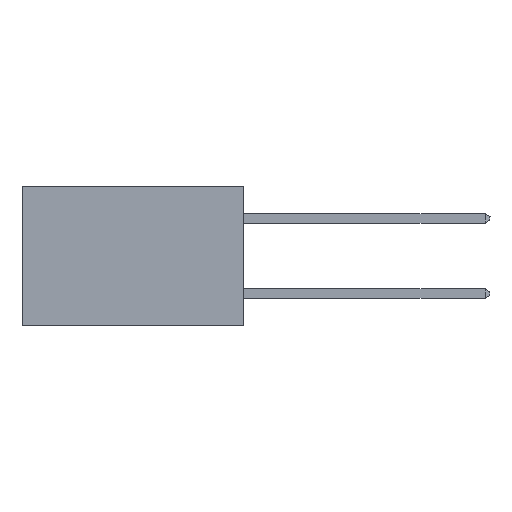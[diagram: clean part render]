
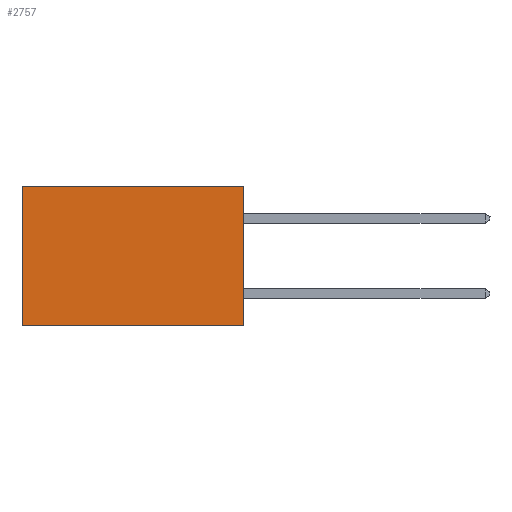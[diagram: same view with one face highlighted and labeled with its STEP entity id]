
A CAD part, left-side view. The second image highlights one B-rep face of the part: STEP entity #2757.
In plain terms, the highlighted planar face has unit normal (-1, 0, 0).
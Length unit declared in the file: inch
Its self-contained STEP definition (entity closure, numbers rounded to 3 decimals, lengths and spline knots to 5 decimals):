
#101 = EDGE_CURVE ( 'NONE', #1082, #926, #6169, .T. ) ;
#853 = LINE ( 'NONE', #5399, #7291 ) ;
#926 = VERTEX_POINT ( 'NONE', #7003 ) ;
#1082 = VERTEX_POINT ( 'NONE', #3588 ) ;
#1115 = AXIS2_PLACEMENT_3D ( 'NONE', #5558, #6310, #5442 ) ;
#1515 = DIRECTION ( 'NONE',  ( 0., 0., -1. ) ) ;
#1756 = EDGE_CURVE ( 'NONE', #5937, #1082, #5213, .T. ) ;
#1921 = EDGE_CURVE ( 'NONE', #5937, #4105, #853, .T. ) ;
#2757 = ADVANCED_FACE ( 'NONE', ( #6491 ), #5560, .F. ) ;
#2960 = VECTOR ( 'NONE', #7861, 39.37008 ) ;
#3369 = CARTESIAN_POINT ( 'NONE',  ( 0.277, 0., -0.37 ) ) ;
#3583 = VECTOR ( 'NONE', #5382, 39.37008 ) ;
#3588 = CARTESIAN_POINT ( 'NONE',  ( 0.277, 0., -0.37 ) ) ;
#3612 = ORIENTED_EDGE ( 'NONE', *, *, #7612, .T. ) ;
#3624 = ORIENTED_EDGE ( 'NONE', *, *, #1756, .F. ) ;
#3842 = ORIENTED_EDGE ( 'NONE', *, *, #101, .F. ) ;
#4047 = ORIENTED_EDGE ( 'NONE', *, *, #1921, .T. ) ;
#4105 = VERTEX_POINT ( 'NONE', #5799 ) ;
#4205 = VECTOR ( 'NONE', #1515, 39.37008 ) ;
#4246 = CARTESIAN_POINT ( 'NONE',  ( 0.277, 0.59, -0.37 ) ) ;
#5026 = DIRECTION ( 'NONE',  ( 0., 1., 0. ) ) ;
#5213 = LINE ( 'NONE', #3369, #3583 ) ;
#5382 = DIRECTION ( 'NONE',  ( 0., 0., -1. ) ) ;
#5399 = CARTESIAN_POINT ( 'NONE',  ( 0.277, 0., 0. ) ) ;
#5442 = DIRECTION ( 'NONE',  ( 0., 0., -1. ) ) ;
#5558 = CARTESIAN_POINT ( 'NONE',  ( 0.277, 0., -0.37 ) ) ;
#5560 = PLANE ( 'NONE',  #1115 ) ;
#5799 = CARTESIAN_POINT ( 'NONE',  ( 0.277, 0.59, 0. ) ) ;
#5937 = VERTEX_POINT ( 'NONE', #6014 ) ;
#6014 = CARTESIAN_POINT ( 'NONE',  ( 0.277, 0., 0. ) ) ;
#6169 = LINE ( 'NONE', #6546, #2960 ) ;
#6310 = DIRECTION ( 'NONE',  ( 1., 0., 0. ) ) ;
#6491 = FACE_OUTER_BOUND ( 'NONE', #7258, .T. ) ;
#6546 = CARTESIAN_POINT ( 'NONE',  ( 0.277, 0., -0.37 ) ) ;
#7003 = CARTESIAN_POINT ( 'NONE',  ( 0.277, 0.59, -0.37 ) ) ;
#7239 = LINE ( 'NONE', #4246, #4205 ) ;
#7258 = EDGE_LOOP ( 'NONE', ( #3612, #3842, #3624, #4047 ) ) ;
#7291 = VECTOR ( 'NONE', #5026, 39.37008 ) ;
#7612 = EDGE_CURVE ( 'NONE', #4105, #926, #7239, .T. ) ;
#7861 = DIRECTION ( 'NONE',  ( 0., 1., 0. ) ) ;
